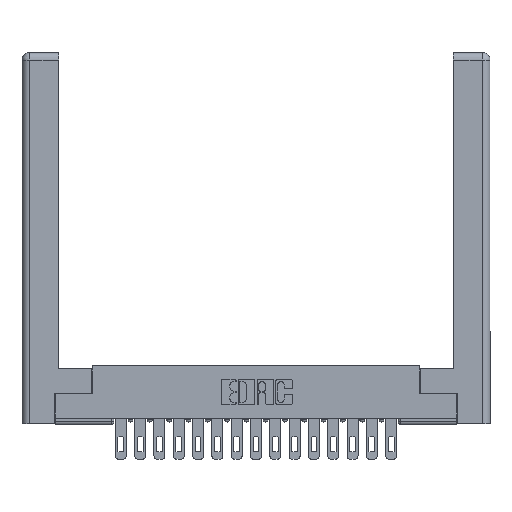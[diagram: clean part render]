
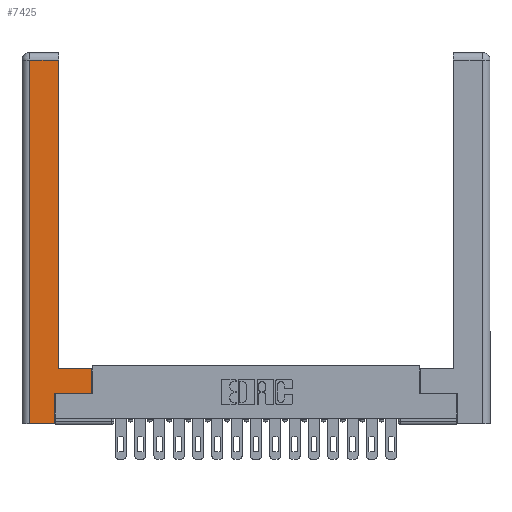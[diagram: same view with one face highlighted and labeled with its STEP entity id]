
A CAD part, top view. The second image highlights one B-rep face of the part: STEP entity #7425.
In plain terms, the highlighted planar face has unit normal (0, 0, 1).
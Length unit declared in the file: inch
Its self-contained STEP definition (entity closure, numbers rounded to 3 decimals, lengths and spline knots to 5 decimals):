
#488 = VERTEX_POINT ( 'NONE', #1071 ) ;
#516 = VECTOR ( 'NONE', #17944, 39.37008 ) ;
#552 = LINE ( 'NONE', #11630, #2170 ) ;
#1071 = CARTESIAN_POINT ( 'NONE',  ( 0.295, 0.45, 0. ) ) ;
#1262 = VERTEX_POINT ( 'NONE', #16621 ) ;
#1628 = CARTESIAN_POINT ( 'NONE',  ( 0.295, 0.45, 0. ) ) ;
#1659 = AXIS2_PLACEMENT_3D ( 'NONE', #18619, #9659, #10165 ) ;
#2025 = EDGE_CURVE ( 'NONE', #19197, #12580, #17964, .T. ) ;
#2143 = EDGE_CURVE ( 'NONE', #1262, #13611, #15430, .T. ) ;
#2170 = VECTOR ( 'NONE', #10250, 39.37008 ) ;
#2778 = CARTESIAN_POINT ( 'NONE',  ( 0.265, 0., 0. ) ) ;
#4168 = VECTOR ( 'NONE', #7330, 39.37008 ) ;
#4555 = VERTEX_POINT ( 'NONE', #9359 ) ;
#6412 = VERTEX_POINT ( 'NONE', #2778 ) ;
#6516 = LINE ( 'NONE', #16281, #10018 ) ;
#6891 = FACE_OUTER_BOUND ( 'NONE', #16002, .T. ) ;
#7151 = ORIENTED_EDGE ( 'NONE', *, *, #17394, .T. ) ;
#7330 = DIRECTION ( 'NONE',  ( 0., 1., 0. ) ) ;
#7425 = ADVANCED_FACE ( 'NONE', ( #6891 ), #18554, .F. ) ;
#7788 = DIRECTION ( 'NONE',  ( 1., 0., 0. ) ) ;
#8222 = LINE ( 'NONE', #9925, #8679 ) ;
#8237 = ORIENTED_EDGE ( 'NONE', *, *, #9622, .T. ) ;
#8525 = ORIENTED_EDGE ( 'NONE', *, *, #10555, .T. ) ;
#8600 = ORIENTED_EDGE ( 'NONE', *, *, #11697, .T. ) ;
#8679 = VECTOR ( 'NONE', #15797, 39.37008 ) ;
#8799 = CARTESIAN_POINT ( 'NONE',  ( 0.0615, 0., 0. ) ) ;
#9062 = DIRECTION ( 'NONE',  ( 0., 1., 0. ) ) ;
#9122 = CARTESIAN_POINT ( 'NONE',  ( 0.565, 0.45, 0. ) ) ;
#9359 = CARTESIAN_POINT ( 'NONE',  ( 0.295, 2.94, 0. ) ) ;
#9622 = EDGE_CURVE ( 'NONE', #4555, #1262, #8222, .T. ) ;
#9641 = CARTESIAN_POINT ( 'NONE',  ( 0.265, 0.245, 0. ) ) ;
#9659 = DIRECTION ( 'NONE',  ( 0., 0., -1. ) ) ;
#9781 = VECTOR ( 'NONE', #16421, 39.37008 ) ;
#9925 = CARTESIAN_POINT ( 'NONE',  ( 0.0615, 2.94, 0. ) ) ;
#9982 = CARTESIAN_POINT ( 'NONE',  ( 0.0615, 0., 0. ) ) ;
#10018 = VECTOR ( 'NONE', #9062, 39.37008 ) ;
#10040 = ORIENTED_EDGE ( 'NONE', *, *, #2025, .T. ) ;
#10165 = DIRECTION ( 'NONE',  ( -1., 0., 0. ) ) ;
#10238 = LINE ( 'NONE', #1628, #9781 ) ;
#10250 = DIRECTION ( 'NONE',  ( 1., 0., 0. ) ) ;
#10528 = EDGE_CURVE ( 'NONE', #488, #4555, #6516, .T. ) ;
#10555 = EDGE_CURVE ( 'NONE', #12580, #488, #10238, .T. ) ;
#11358 = CARTESIAN_POINT ( 'NONE',  ( 0.565, 0.245, 0. ) ) ;
#11473 = VECTOR ( 'NONE', #13032, 39.37008 ) ;
#11630 = CARTESIAN_POINT ( 'NONE',  ( 0.265, 0., 0. ) ) ;
#11697 = EDGE_CURVE ( 'NONE', #6412, #13409, #19286, .T. ) ;
#12126 = ORIENTED_EDGE ( 'NONE', *, *, #18968, .T. ) ;
#12192 = CARTESIAN_POINT ( 'NONE',  ( 0.565, 0.245, 0. ) ) ;
#12580 = VERTEX_POINT ( 'NONE', #17916 ) ;
#12585 = ORIENTED_EDGE ( 'NONE', *, *, #10528, .T. ) ;
#13032 = DIRECTION ( 'NONE',  ( 0., -1., 0. ) ) ;
#13057 = LINE ( 'NONE', #12192, #16323 ) ;
#13213 = ORIENTED_EDGE ( 'NONE', *, *, #2143, .T. ) ;
#13409 = VERTEX_POINT ( 'NONE', #9641 ) ;
#13611 = VERTEX_POINT ( 'NONE', #8799 ) ;
#14743 = CARTESIAN_POINT ( 'NONE',  ( 0.265, 0.245, 0. ) ) ;
#15430 = LINE ( 'NONE', #9982, #11473 ) ;
#15797 = DIRECTION ( 'NONE',  ( -1., 0., 0. ) ) ;
#16002 = EDGE_LOOP ( 'NONE', ( #12585, #8237, #13213, #7151, #8600, #12126, #10040, #8525 ) ) ;
#16281 = CARTESIAN_POINT ( 'NONE',  ( 0.295, 3., 0. ) ) ;
#16323 = VECTOR ( 'NONE', #7788, 39.37008 ) ;
#16421 = DIRECTION ( 'NONE',  ( -1., 0., 0. ) ) ;
#16621 = CARTESIAN_POINT ( 'NONE',  ( 0.0615, 2.94, 0. ) ) ;
#17394 = EDGE_CURVE ( 'NONE', #13611, #6412, #552, .T. ) ;
#17916 = CARTESIAN_POINT ( 'NONE',  ( 0.565, 0.45, 0. ) ) ;
#17944 = DIRECTION ( 'NONE',  ( 0., 1., 0. ) ) ;
#17964 = LINE ( 'NONE', #9122, #516 ) ;
#18554 = PLANE ( 'NONE',  #1659 ) ;
#18619 = CARTESIAN_POINT ( 'NONE',  ( 0., 0., 0. ) ) ;
#18968 = EDGE_CURVE ( 'NONE', #13409, #19197, #13057, .T. ) ;
#19197 = VERTEX_POINT ( 'NONE', #11358 ) ;
#19286 = LINE ( 'NONE', #14743, #4168 ) ;
